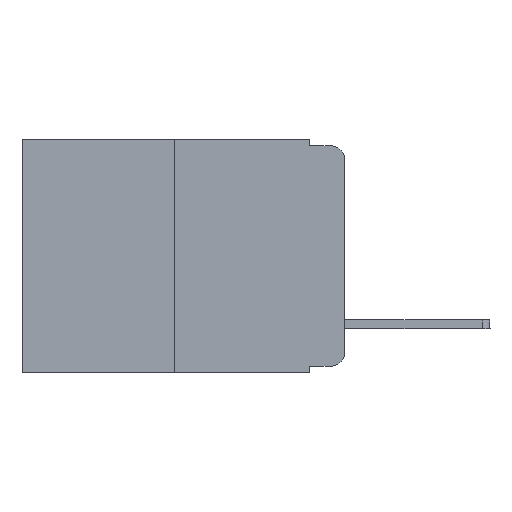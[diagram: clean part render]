
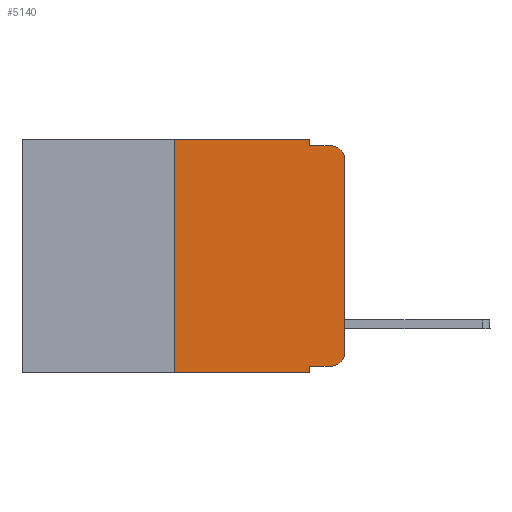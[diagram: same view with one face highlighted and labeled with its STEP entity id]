
A CAD part, left-side view. The second image highlights one B-rep face of the part: STEP entity #5140.
In plain terms, the highlighted planar face has unit normal (-1, 0, 0).
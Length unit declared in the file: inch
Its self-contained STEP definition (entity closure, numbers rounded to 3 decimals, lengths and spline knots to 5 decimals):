
#288 = DIRECTION ( 'NONE',  ( 0., -1., 0. ) ) ;
#906 = EDGE_CURVE ( 'NONE', #6836, #11649, #11796, .T. ) ;
#1095 = DIRECTION ( 'NONE',  ( -1., 0., 0. ) ) ;
#1190 = AXIS2_PLACEMENT_3D ( 'NONE', #15244, #7240, #1896 ) ;
#1270 = CARTESIAN_POINT ( 'NONE',  ( 0., 0.473, -0.343 ) ) ;
#1345 = ORIENTED_EDGE ( 'NONE', *, *, #7478, .F. ) ;
#1703 = CARTESIAN_POINT ( 'NONE',  ( 0., 0.473, 0. ) ) ;
#1764 = CARTESIAN_POINT ( 'NONE',  ( 0., 0.25, 0. ) ) ;
#1770 = PLANE ( 'NONE',  #11301 ) ;
#1772 = DIRECTION ( 'NONE',  ( 0., -1., 0. ) ) ;
#1846 = EDGE_CURVE ( 'NONE', #11649, #6644, #12388, .T. ) ;
#1896 = DIRECTION ( 'NONE',  ( 0., 0., -1. ) ) ;
#1970 = DIRECTION ( 'NONE',  ( 0., 0., -1. ) ) ;
#1989 = DIRECTION ( 'NONE',  ( 0., 0., -1. ) ) ;
#2425 = DIRECTION ( 'NONE',  ( 0., 0., -1. ) ) ;
#2535 = LINE ( 'NONE', #6269, #9886 ) ;
#2623 = CARTESIAN_POINT ( 'NONE',  ( 0., 0.051, -0.343 ) ) ;
#3239 = CARTESIAN_POINT ( 'NONE',  ( 0., 0., -0.313 ) ) ;
#3339 = CARTESIAN_POINT ( 'NONE',  ( 0., 0.051, 0. ) ) ;
#3349 = LINE ( 'NONE', #10812, #7131 ) ;
#3439 = VECTOR ( 'NONE', #11871, 39.37008 ) ;
#4097 = CARTESIAN_POINT ( 'NONE',  ( 0., 0., 0. ) ) ;
#4279 = EDGE_CURVE ( 'NONE', #15621, #6836, #8351, .T. ) ;
#4444 = LINE ( 'NONE', #5956, #14307 ) ;
#4580 = DIRECTION ( 'NONE',  ( 0., 0., -1. ) ) ;
#4982 = CARTESIAN_POINT ( 'NONE',  ( 0., 0.051, -0.01 ) ) ;
#5140 = ADVANCED_FACE ( 'NONE', ( #14211 ), #1770, .F. ) ;
#5478 = ORIENTED_EDGE ( 'NONE', *, *, #17003, .T. ) ;
#5574 = VERTEX_POINT ( 'NONE', #15494 ) ;
#5718 = LINE ( 'NONE', #1270, #13854 ) ;
#5956 = CARTESIAN_POINT ( 'NONE',  ( 0., 0.473, 0. ) ) ;
#6269 = CARTESIAN_POINT ( 'NONE',  ( 0., 0.051, -0.01 ) ) ;
#6429 = VERTEX_POINT ( 'NONE', #4982 ) ;
#6644 = VERTEX_POINT ( 'NONE', #6895 ) ;
#6836 = VERTEX_POINT ( 'NONE', #3239 ) ;
#6895 = CARTESIAN_POINT ( 'NONE',  ( 0., 0.02, -0.01 ) ) ;
#6922 = EDGE_CURVE ( 'NONE', #6429, #6644, #2535, .T. ) ;
#7042 = CARTESIAN_POINT ( 'NONE',  ( 0., 0.25, -0.343 ) ) ;
#7131 = VECTOR ( 'NONE', #288, 39.37008 ) ;
#7203 = LINE ( 'NONE', #1764, #13230 ) ;
#7240 = DIRECTION ( 'NONE',  ( -1., 0., 0. ) ) ;
#7435 = VERTEX_POINT ( 'NONE', #9266 ) ;
#7447 = ORIENTED_EDGE ( 'NONE', *, *, #6922, .F. ) ;
#7473 = VECTOR ( 'NONE', #1970, 39.37008 ) ;
#7478 = EDGE_CURVE ( 'NONE', #5574, #7435, #4444, .T. ) ;
#8174 = DIRECTION ( 'NONE',  ( 0., -1., 0. ) ) ;
#8351 = CIRCLE ( 'NONE', #1190, 0.02 ) ;
#8618 = DIRECTION ( 'NONE',  ( 1., 0., 0. ) ) ;
#8925 = EDGE_CURVE ( 'NONE', #11938, #16827, #16738, .T. ) ;
#9266 = CARTESIAN_POINT ( 'NONE',  ( 0., 0.051, 0. ) ) ;
#9389 = ORIENTED_EDGE ( 'NONE', *, *, #8925, .F. ) ;
#9886 = VECTOR ( 'NONE', #13020, 39.37008 ) ;
#10043 = CARTESIAN_POINT ( 'NONE',  ( 0., 0., -0.03 ) ) ;
#10270 = AXIS2_PLACEMENT_3D ( 'NONE', #17073, #1095, #2425 ) ;
#10776 = EDGE_CURVE ( 'NONE', #7435, #6429, #12907, .T. ) ;
#10812 = CARTESIAN_POINT ( 'NONE',  ( 0., 0.051, -0.333 ) ) ;
#10865 = VECTOR ( 'NONE', #1989, 39.37008 ) ;
#11301 = AXIS2_PLACEMENT_3D ( 'NONE', #1703, #8618, #4580 ) ;
#11649 = VERTEX_POINT ( 'NONE', #10043 ) ;
#11673 = ORIENTED_EDGE ( 'NONE', *, *, #4279, .T. ) ;
#11679 = EDGE_CURVE ( 'NONE', #17105, #5574, #7203, .T. ) ;
#11796 = LINE ( 'NONE', #4097, #3439 ) ;
#11871 = DIRECTION ( 'NONE',  ( 0., 0., 1. ) ) ;
#11938 = VERTEX_POINT ( 'NONE', #14106 ) ;
#12061 = ORIENTED_EDGE ( 'NONE', *, *, #11679, .F. ) ;
#12155 = ORIENTED_EDGE ( 'NONE', *, *, #906, .T. ) ;
#12388 = CIRCLE ( 'NONE', #10270, 0.02 ) ;
#12463 = DIRECTION ( 'NONE',  ( 0., 0., 1. ) ) ;
#12907 = LINE ( 'NONE', #14028, #7473 ) ;
#13020 = DIRECTION ( 'NONE',  ( 0., -1., 0. ) ) ;
#13230 = VECTOR ( 'NONE', #12463, 39.37008 ) ;
#13280 = ORIENTED_EDGE ( 'NONE', *, *, #15667, .T. ) ;
#13854 = VECTOR ( 'NONE', #8174, 39.37008 ) ;
#14028 = CARTESIAN_POINT ( 'NONE',  ( 0., 0.051, 0. ) ) ;
#14106 = CARTESIAN_POINT ( 'NONE',  ( 0., 0.051, -0.333 ) ) ;
#14211 = FACE_OUTER_BOUND ( 'NONE', #17235, .T. ) ;
#14307 = VECTOR ( 'NONE', #1772, 39.37008 ) ;
#14371 = ORIENTED_EDGE ( 'NONE', *, *, #10776, .F. ) ;
#15244 = CARTESIAN_POINT ( 'NONE',  ( 0., 0.02, -0.313 ) ) ;
#15494 = CARTESIAN_POINT ( 'NONE',  ( 0., 0.25, 0. ) ) ;
#15621 = VERTEX_POINT ( 'NONE', #16319 ) ;
#15667 = EDGE_CURVE ( 'NONE', #17105, #16827, #5718, .T. ) ;
#16319 = CARTESIAN_POINT ( 'NONE',  ( 0., 0.02, -0.333 ) ) ;
#16386 = ORIENTED_EDGE ( 'NONE', *, *, #1846, .T. ) ;
#16738 = LINE ( 'NONE', #3339, #10865 ) ;
#16827 = VERTEX_POINT ( 'NONE', #2623 ) ;
#17003 = EDGE_CURVE ( 'NONE', #11938, #15621, #3349, .T. ) ;
#17073 = CARTESIAN_POINT ( 'NONE',  ( 0., 0.02, -0.03 ) ) ;
#17105 = VERTEX_POINT ( 'NONE', #7042 ) ;
#17235 = EDGE_LOOP ( 'NONE', ( #12155, #16386, #7447, #14371, #1345, #12061, #13280, #9389, #5478, #11673 ) ) ;
